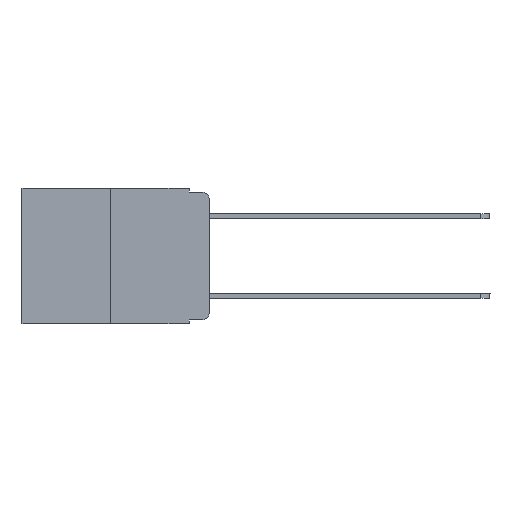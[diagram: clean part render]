
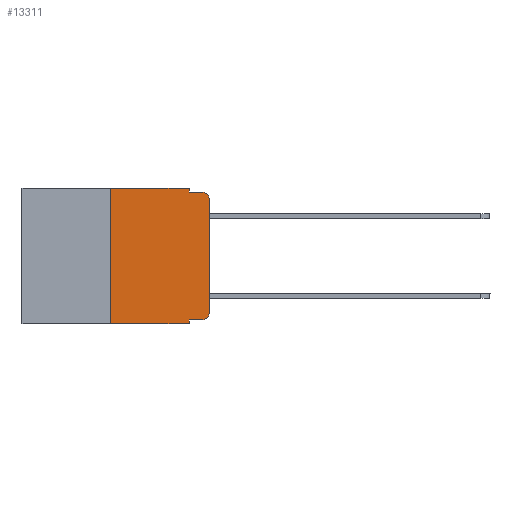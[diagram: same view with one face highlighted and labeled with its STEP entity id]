
A CAD part, left-side view. The second image highlights one B-rep face of the part: STEP entity #13311.
In plain terms, the highlighted planar face has unit normal (-1, 0, 0).
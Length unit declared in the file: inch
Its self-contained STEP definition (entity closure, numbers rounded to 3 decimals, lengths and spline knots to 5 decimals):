
#94 = VECTOR ( 'NONE', #1449, 39.37008 ) ;
#105 = VERTEX_POINT ( 'NONE', #12364 ) ;
#121 = LINE ( 'NONE', #6615, #7398 ) ;
#185 = LINE ( 'NONE', #4493, #2040 ) ;
#189 = CARTESIAN_POINT ( 'NONE',  ( 0., 0.25, -0.343 ) ) ;
#314 = CARTESIAN_POINT ( 'NONE',  ( 0., 0.051, -0.01 ) ) ;
#931 = EDGE_CURVE ( 'NONE', #9029, #7838, #2379, .T. ) ;
#950 = VERTEX_POINT ( 'NONE', #1389 ) ;
#996 = ORIENTED_EDGE ( 'NONE', *, *, #931, .F. ) ;
#1015 = VECTOR ( 'NONE', #10339, 39.37008 ) ;
#1127 = FACE_OUTER_BOUND ( 'NONE', #4546, .T. ) ;
#1269 = VECTOR ( 'NONE', #4603, 39.37008 ) ;
#1276 = CARTESIAN_POINT ( 'NONE',  ( 0., 0.051, 0. ) ) ;
#1389 = CARTESIAN_POINT ( 'NONE',  ( 0., 0.051, 0. ) ) ;
#1449 = DIRECTION ( 'NONE',  ( 0., 0., -1. ) ) ;
#1573 = VECTOR ( 'NONE', #4734, 39.37008 ) ;
#1621 = VERTEX_POINT ( 'NONE', #4158 ) ;
#1978 = VERTEX_POINT ( 'NONE', #4840 ) ;
#2019 = CARTESIAN_POINT ( 'NONE',  ( 0., 0.051, -0.333 ) ) ;
#2040 = VECTOR ( 'NONE', #6748, 39.37008 ) ;
#2191 = ORIENTED_EDGE ( 'NONE', *, *, #3056, .T. ) ;
#2379 = LINE ( 'NONE', #9018, #94 ) ;
#3036 = AXIS2_PLACEMENT_3D ( 'NONE', #9275, #13595, #8188 ) ;
#3044 = CARTESIAN_POINT ( 'NONE',  ( 0., 0.25, 0. ) ) ;
#3056 = EDGE_CURVE ( 'NONE', #9636, #1621, #12005, .T. ) ;
#3510 = DIRECTION ( 'NONE',  ( 0., -1., 0. ) ) ;
#3761 = CARTESIAN_POINT ( 'NONE',  ( 0., 0.473, -0.343 ) ) ;
#4158 = CARTESIAN_POINT ( 'NONE',  ( 0., 0., -0.313 ) ) ;
#4352 = PLANE ( 'NONE',  #10394 ) ;
#4493 = CARTESIAN_POINT ( 'NONE',  ( 0., 0.051, -0.333 ) ) ;
#4546 = EDGE_LOOP ( 'NONE', ( #11771, #7053, #7305, #9789, #5747, #11636, #13571, #996, #6898, #2191 ) ) ;
#4603 = DIRECTION ( 'NONE',  ( 0., -1., 0. ) ) ;
#4734 = DIRECTION ( 'NONE',  ( 0., -1., 0. ) ) ;
#4790 = VECTOR ( 'NONE', #3510, 39.37008 ) ;
#4840 = CARTESIAN_POINT ( 'NONE',  ( 0., 0.02, -0.01 ) ) ;
#5598 = LINE ( 'NONE', #9949, #1573 ) ;
#5747 = ORIENTED_EDGE ( 'NONE', *, *, #13046, .F. ) ;
#5757 = DIRECTION ( 'NONE',  ( 0., 0., 1. ) ) ;
#5821 = EDGE_CURVE ( 'NONE', #11378, #7838, #5946, .T. ) ;
#5850 = EDGE_CURVE ( 'NONE', #9029, #9636, #185, .T. ) ;
#5946 = LINE ( 'NONE', #3761, #4790 ) ;
#6462 = EDGE_CURVE ( 'NONE', #11378, #11651, #11530, .T. ) ;
#6554 = DIRECTION ( 'NONE',  ( 0., 0., -1. ) ) ;
#6615 = CARTESIAN_POINT ( 'NONE',  ( 0., 0., 0. ) ) ;
#6655 = VERTEX_POINT ( 'NONE', #12228 ) ;
#6748 = DIRECTION ( 'NONE',  ( 0., -1., 0. ) ) ;
#6898 = ORIENTED_EDGE ( 'NONE', *, *, #5850, .T. ) ;
#7053 = ORIENTED_EDGE ( 'NONE', *, *, #8151, .T. ) ;
#7305 = ORIENTED_EDGE ( 'NONE', *, *, #7542, .F. ) ;
#7398 = VECTOR ( 'NONE', #5757, 39.37008 ) ;
#7415 = LINE ( 'NONE', #1276, #12971 ) ;
#7542 = EDGE_CURVE ( 'NONE', #6655, #1978, #13191, .T. ) ;
#7838 = VERTEX_POINT ( 'NONE', #9129 ) ;
#8151 = EDGE_CURVE ( 'NONE', #105, #1978, #9150, .T. ) ;
#8188 = DIRECTION ( 'NONE',  ( 0., 0., -1. ) ) ;
#8208 = EDGE_CURVE ( 'NONE', #950, #6655, #7415, .T. ) ;
#8651 = CARTESIAN_POINT ( 'NONE',  ( 0., 0.25, 0. ) ) ;
#8665 = CARTESIAN_POINT ( 'NONE',  ( 0., 0.473, 0. ) ) ;
#9018 = CARTESIAN_POINT ( 'NONE',  ( 0., 0.051, 0. ) ) ;
#9029 = VERTEX_POINT ( 'NONE', #2019 ) ;
#9129 = CARTESIAN_POINT ( 'NONE',  ( 0., 0.051, -0.343 ) ) ;
#9150 = CIRCLE ( 'NONE', #3036, 0.02 ) ;
#9178 = DIRECTION ( 'NONE',  ( 1., 0., 0. ) ) ;
#9275 = CARTESIAN_POINT ( 'NONE',  ( 0., 0.02, -0.03 ) ) ;
#9636 = VERTEX_POINT ( 'NONE', #11132 ) ;
#9789 = ORIENTED_EDGE ( 'NONE', *, *, #8208, .F. ) ;
#9915 = DIRECTION ( 'NONE',  ( 0., 0., -1. ) ) ;
#9949 = CARTESIAN_POINT ( 'NONE',  ( 0., 0.473, 0. ) ) ;
#9978 = CARTESIAN_POINT ( 'NONE',  ( 0., 0.02, -0.313 ) ) ;
#10339 = DIRECTION ( 'NONE',  ( 0., 0., 1. ) ) ;
#10394 = AXIS2_PLACEMENT_3D ( 'NONE', #8665, #9178, #13414 ) ;
#11132 = CARTESIAN_POINT ( 'NONE',  ( 0., 0.02, -0.333 ) ) ;
#11378 = VERTEX_POINT ( 'NONE', #189 ) ;
#11413 = EDGE_CURVE ( 'NONE', #1621, #105, #121, .T. ) ;
#11530 = LINE ( 'NONE', #3044, #1015 ) ;
#11636 = ORIENTED_EDGE ( 'NONE', *, *, #6462, .F. ) ;
#11651 = VERTEX_POINT ( 'NONE', #8651 ) ;
#11771 = ORIENTED_EDGE ( 'NONE', *, *, #11413, .T. ) ;
#12005 = CIRCLE ( 'NONE', #13133, 0.02 ) ;
#12089 = DIRECTION ( 'NONE',  ( -1., 0., 0. ) ) ;
#12228 = CARTESIAN_POINT ( 'NONE',  ( 0., 0.051, -0.01 ) ) ;
#12364 = CARTESIAN_POINT ( 'NONE',  ( 0., 0., -0.03 ) ) ;
#12971 = VECTOR ( 'NONE', #6554, 39.37008 ) ;
#13046 = EDGE_CURVE ( 'NONE', #11651, #950, #5598, .T. ) ;
#13133 = AXIS2_PLACEMENT_3D ( 'NONE', #9978, #12089, #9915 ) ;
#13191 = LINE ( 'NONE', #314, #1269 ) ;
#13311 = ADVANCED_FACE ( 'NONE', ( #1127 ), #4352, .F. ) ;
#13414 = DIRECTION ( 'NONE',  ( 0., 0., -1. ) ) ;
#13571 = ORIENTED_EDGE ( 'NONE', *, *, #5821, .T. ) ;
#13595 = DIRECTION ( 'NONE',  ( -1., 0., 0. ) ) ;
